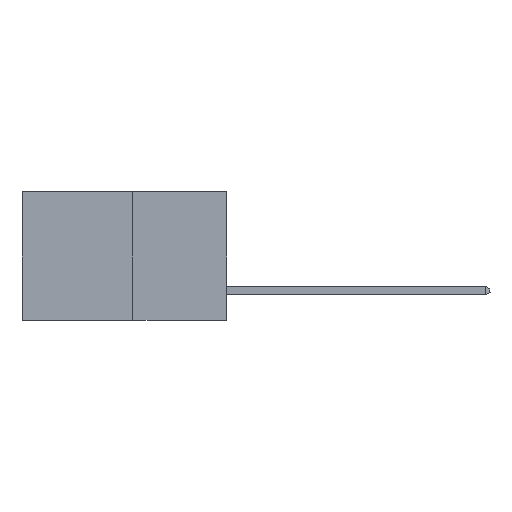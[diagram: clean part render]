
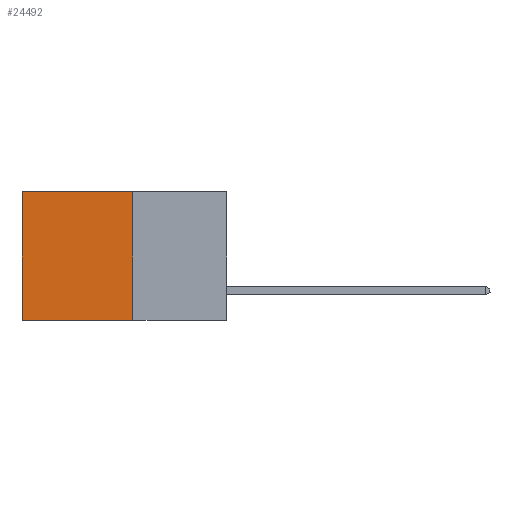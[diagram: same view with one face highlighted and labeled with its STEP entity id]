
A CAD part, left-side view. The second image highlights one B-rep face of the part: STEP entity #24492.
In plain terms, the highlighted planar face has unit normal (-1, 0, 0).
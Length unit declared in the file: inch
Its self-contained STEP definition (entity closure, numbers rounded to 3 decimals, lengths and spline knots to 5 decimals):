
#760 = ORIENTED_EDGE ( 'NONE', *, *, #8325, .T. ) ;
#1403 = DIRECTION ( 'NONE',  ( 0., 0., -1. ) ) ;
#1495 = CARTESIAN_POINT ( 'NONE',  ( 0.277, 0.59, 0. ) ) ;
#1799 = VERTEX_POINT ( 'NONE', #11300 ) ;
#2000 = EDGE_LOOP ( 'NONE', ( #21260, #29891, #27065, #760 ) ) ;
#4049 = EDGE_CURVE ( 'NONE', #1799, #13306, #24239, .T. ) ;
#6553 = CARTESIAN_POINT ( 'NONE',  ( 0.277, 0.59, -0.37 ) ) ;
#7274 = VERTEX_POINT ( 'NONE', #6553 ) ;
#8325 = EDGE_CURVE ( 'NONE', #1799, #20317, #22289, .T. ) ;
#8878 = CARTESIAN_POINT ( 'NONE',  ( 0.277, 0.27, -0.37 ) ) ;
#11300 = CARTESIAN_POINT ( 'NONE',  ( 0.277, 0.27, 0. ) ) ;
#11517 = VECTOR ( 'NONE', #15776, 39.37008 ) ;
#13166 = CARTESIAN_POINT ( 'NONE',  ( 0.277, 0.27, -0.37 ) ) ;
#13306 = VERTEX_POINT ( 'NONE', #19188 ) ;
#13362 = CARTESIAN_POINT ( 'NONE',  ( 0.277, 0.59, -0.37 ) ) ;
#14773 = VECTOR ( 'NONE', #25396, 39.37008 ) ;
#15219 = AXIS2_PLACEMENT_3D ( 'NONE', #13166, #15600, #1403 ) ;
#15600 = DIRECTION ( 'NONE',  ( 1., 0., 0. ) ) ;
#15776 = DIRECTION ( 'NONE',  ( 0., 0., -1. ) ) ;
#16371 = CARTESIAN_POINT ( 'NONE',  ( 0.277, 0.27, -0.37 ) ) ;
#17022 = DIRECTION ( 'NONE',  ( 0., 0., -1. ) ) ;
#17886 = EDGE_CURVE ( 'NONE', #20317, #7274, #19329, .T. ) ;
#19188 = CARTESIAN_POINT ( 'NONE',  ( 0.277, 0.27, -0.37 ) ) ;
#19309 = EDGE_CURVE ( 'NONE', #13306, #7274, #27323, .T. ) ;
#19329 = LINE ( 'NONE', #13362, #11517 ) ;
#20317 = VERTEX_POINT ( 'NONE', #1495 ) ;
#21260 = ORIENTED_EDGE ( 'NONE', *, *, #17886, .T. ) ;
#22289 = LINE ( 'NONE', #27260, #29240 ) ;
#22651 = DIRECTION ( 'NONE',  ( 0., 1., 0. ) ) ;
#23517 = VECTOR ( 'NONE', #17022, 39.37008 ) ;
#24239 = LINE ( 'NONE', #16371, #23517 ) ;
#24492 = ADVANCED_FACE ( 'NONE', ( #28015 ), #27349, .F. ) ;
#25396 = DIRECTION ( 'NONE',  ( 0., 1., 0. ) ) ;
#27065 = ORIENTED_EDGE ( 'NONE', *, *, #4049, .F. ) ;
#27260 = CARTESIAN_POINT ( 'NONE',  ( 0.277, 0.27, 0. ) ) ;
#27323 = LINE ( 'NONE', #8878, #14773 ) ;
#27349 = PLANE ( 'NONE',  #15219 ) ;
#28015 = FACE_OUTER_BOUND ( 'NONE', #2000, .T. ) ;
#29240 = VECTOR ( 'NONE', #22651, 39.37008 ) ;
#29891 = ORIENTED_EDGE ( 'NONE', *, *, #19309, .F. ) ;
